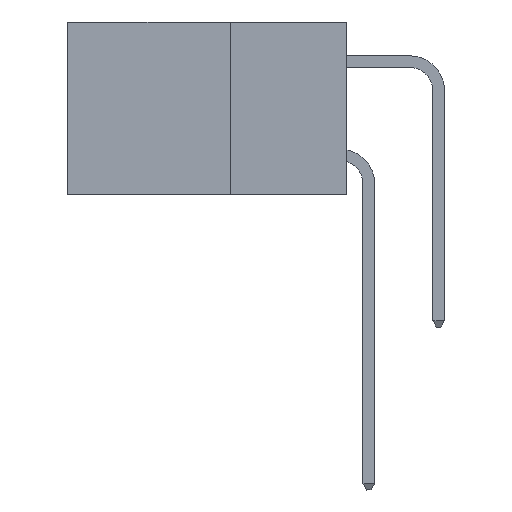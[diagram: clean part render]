
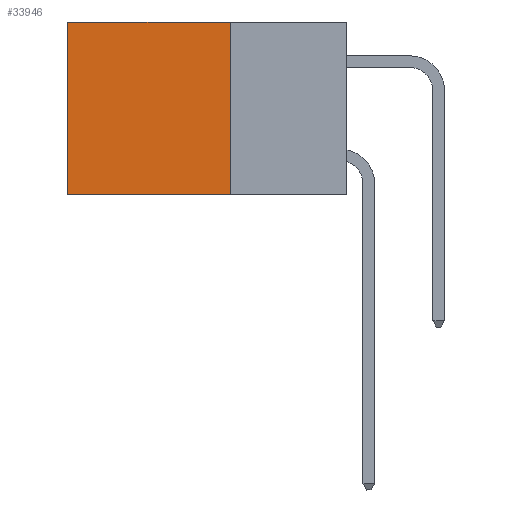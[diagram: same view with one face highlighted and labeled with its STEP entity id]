
A CAD part, left-side view. The second image highlights one B-rep face of the part: STEP entity #33946.
In plain terms, the highlighted planar face has unit normal (-1, 0, 0).
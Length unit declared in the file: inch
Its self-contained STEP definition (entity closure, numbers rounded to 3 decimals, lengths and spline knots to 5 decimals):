
#989 = LINE ( 'NONE', #8651, #20578 ) ;
#3159 = CARTESIAN_POINT ( 'NONE',  ( 0.2875, 0.25, 0. ) ) ;
#3700 = DIRECTION ( 'NONE',  ( 0., 0., -1. ) ) ;
#3800 = EDGE_CURVE ( 'NONE', #38319, #18686, #25585, .T. ) ;
#4307 = VECTOR ( 'NONE', #14379, 39.37008 ) ;
#4947 = FACE_OUTER_BOUND ( 'NONE', #11345, .T. ) ;
#5077 = EDGE_CURVE ( 'NONE', #33491, #34126, #32531, .T. ) ;
#8651 = CARTESIAN_POINT ( 'NONE',  ( 0.2875, 0.6, 0. ) ) ;
#8723 = LINE ( 'NONE', #20939, #4307 ) ;
#11142 = EDGE_CURVE ( 'NONE', #18686, #34126, #989, .T. ) ;
#11345 = EDGE_LOOP ( 'NONE', ( #15188, #31758, #24351, #20832 ) ) ;
#14379 = DIRECTION ( 'NONE',  ( 0., 0., -1. ) ) ;
#15188 = ORIENTED_EDGE ( 'NONE', *, *, #11142, .T. ) ;
#15225 = DIRECTION ( 'NONE',  ( 0., 1., 0. ) ) ;
#15795 = DIRECTION ( 'NONE',  ( 1., 0., 0. ) ) ;
#16415 = CARTESIAN_POINT ( 'NONE',  ( 0.2875, 0.25, -0.37 ) ) ;
#17293 = VECTOR ( 'NONE', #15225, 39.37008 ) ;
#18686 = VERTEX_POINT ( 'NONE', #30400 ) ;
#19216 = PLANE ( 'NONE',  #25665 ) ;
#20578 = VECTOR ( 'NONE', #27669, 39.37008 ) ;
#20815 = VECTOR ( 'NONE', #36394, 39.37008 ) ;
#20832 = ORIENTED_EDGE ( 'NONE', *, *, #3800, .T. ) ;
#20939 = CARTESIAN_POINT ( 'NONE',  ( 0.2875, 0.25, 0. ) ) ;
#23258 = CARTESIAN_POINT ( 'NONE',  ( 0.2875, 0.6, -0.37 ) ) ;
#24351 = ORIENTED_EDGE ( 'NONE', *, *, #36857, .F. ) ;
#24403 = CARTESIAN_POINT ( 'NONE',  ( 0.2875, 0.25, -0.37 ) ) ;
#25585 = LINE ( 'NONE', #27769, #17293 ) ;
#25665 = AXIS2_PLACEMENT_3D ( 'NONE', #3159, #15795, #3700 ) ;
#27669 = DIRECTION ( 'NONE',  ( 0., 0., -1. ) ) ;
#27769 = CARTESIAN_POINT ( 'NONE',  ( 0.2875, 0.25, 0. ) ) ;
#30400 = CARTESIAN_POINT ( 'NONE',  ( 0.2875, 0.6, 0. ) ) ;
#31758 = ORIENTED_EDGE ( 'NONE', *, *, #5077, .F. ) ;
#32531 = LINE ( 'NONE', #24403, #20815 ) ;
#33491 = VERTEX_POINT ( 'NONE', #16415 ) ;
#33946 = ADVANCED_FACE ( 'NONE', ( #4947 ), #19216, .F. ) ;
#34126 = VERTEX_POINT ( 'NONE', #23258 ) ;
#36394 = DIRECTION ( 'NONE',  ( 0., 1., 0. ) ) ;
#36857 = EDGE_CURVE ( 'NONE', #38319, #33491, #8723, .T. ) ;
#38319 = VERTEX_POINT ( 'NONE', #40008 ) ;
#40008 = CARTESIAN_POINT ( 'NONE',  ( 0.2875, 0.25, 0. ) ) ;
